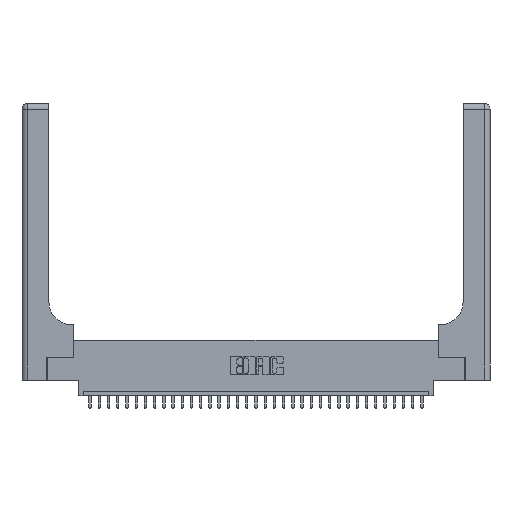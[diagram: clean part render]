
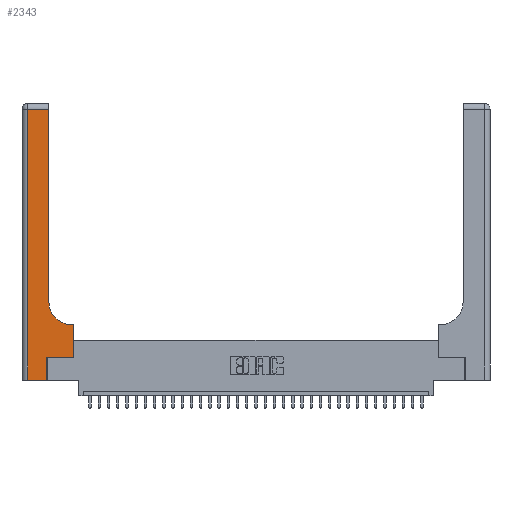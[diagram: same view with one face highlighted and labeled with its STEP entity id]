
A CAD part, top view. The second image highlights one B-rep face of the part: STEP entity #2343.
In plain terms, the highlighted planar face has unit normal (0, 0, 1).
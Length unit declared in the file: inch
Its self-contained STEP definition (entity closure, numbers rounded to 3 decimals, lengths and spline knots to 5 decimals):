
#44 = DIRECTION ( 'NONE',  ( 1., 0., 0. ) ) ;
#453 = CARTESIAN_POINT ( 'NONE',  ( 0.2915, 0.6, 0.37 ) ) ;
#1521 = CARTESIAN_POINT ( 'NONE',  ( 0.5415, 0.85, 0.37 ) ) ;
#1815 = CARTESIAN_POINT ( 'NONE',  ( 0.06, 0., 0.37 ) ) ;
#1894 = DIRECTION ( 'NONE',  ( -1., 0., 0. ) ) ;
#2343 = ADVANCED_FACE ( 'NONE', ( #16079 ), #14926, .F. ) ;
#3345 = LINE ( 'NONE', #25797, #30321 ) ;
#5041 = VECTOR ( 'NONE', #14339, 39.37008 ) ;
#7124 = CARTESIAN_POINT ( 'NONE',  ( 0., 3., 0.37 ) ) ;
#7557 = CARTESIAN_POINT ( 'NONE',  ( 0.06, 3., 0.37 ) ) ;
#7949 = CARTESIAN_POINT ( 'NONE',  ( 0.269, 0., 0.37 ) ) ;
#8164 = EDGE_CURVE ( 'NONE', #15728, #21541, #27175, .T. ) ;
#8396 = CARTESIAN_POINT ( 'NONE',  ( 0.2915, 0.85, 0.37 ) ) ;
#10462 = AXIS2_PLACEMENT_3D ( 'NONE', #1521, #33048, #30664 ) ;
#10763 = EDGE_CURVE ( 'NONE', #21541, #19920, #27013, .T. ) ;
#11228 = EDGE_LOOP ( 'NONE', ( #24741, #26455, #27806, #13317, #22384, #18113, #16411, #21456, #15497 ) ) ;
#11329 = DIRECTION ( 'NONE',  ( -1., 0., 0. ) ) ;
#11653 = VERTEX_POINT ( 'NONE', #29360 ) ;
#12967 = VECTOR ( 'NONE', #33252, 39.37008 ) ;
#13317 = ORIENTED_EDGE ( 'NONE', *, *, #8164, .T. ) ;
#14166 = CARTESIAN_POINT ( 'NONE',  ( 0.5415, 0.6, 0.37 ) ) ;
#14339 = DIRECTION ( 'NONE',  ( 1., 0., 0. ) ) ;
#14682 = VECTOR ( 'NONE', #11329, 39.37008 ) ;
#14926 = PLANE ( 'NONE',  #19494 ) ;
#15497 = ORIENTED_EDGE ( 'NONE', *, *, #32342, .T. ) ;
#15711 = DIRECTION ( 'NONE',  ( 0., -1., 0. ) ) ;
#15728 = VERTEX_POINT ( 'NONE', #1815 ) ;
#15775 = VECTOR ( 'NONE', #33637, 39.37008 ) ;
#16079 = FACE_OUTER_BOUND ( 'NONE', #11228, .T. ) ;
#16411 = ORIENTED_EDGE ( 'NONE', *, *, #29779, .T. ) ;
#16461 = EDGE_CURVE ( 'NONE', #25185, #27807, #3345, .T. ) ;
#16769 = VECTOR ( 'NONE', #26402, 39.37008 ) ;
#17730 = CARTESIAN_POINT ( 'NONE',  ( 0.269, 0., 0.37 ) ) ;
#18113 = ORIENTED_EDGE ( 'NONE', *, *, #22269, .T. ) ;
#18917 = VERTEX_POINT ( 'NONE', #21245 ) ;
#18991 = LINE ( 'NONE', #27727, #5041 ) ;
#19330 = EDGE_CURVE ( 'NONE', #29041, #15728, #31767, .T. ) ;
#19358 = CIRCLE ( 'NONE', #10462, 0.25 ) ;
#19494 = AXIS2_PLACEMENT_3D ( 'NONE', #7124, #27985, #1894 ) ;
#19920 = VERTEX_POINT ( 'NONE', #25752 ) ;
#20767 = CARTESIAN_POINT ( 'NONE',  ( 0., 0., 0.37 ) ) ;
#21245 = CARTESIAN_POINT ( 'NONE',  ( 0.5585, 0.25, 0.37 ) ) ;
#21456 = ORIENTED_EDGE ( 'NONE', *, *, #29005, .T. ) ;
#21541 = VERTEX_POINT ( 'NONE', #7949 ) ;
#21593 = LINE ( 'NONE', #28043, #12967 ) ;
#22269 = EDGE_CURVE ( 'NONE', #19920, #18917, #18991, .T. ) ;
#22275 = VECTOR ( 'NONE', #44, 39.37008 ) ;
#22384 = ORIENTED_EDGE ( 'NONE', *, *, #10763, .T. ) ;
#22722 = LINE ( 'NONE', #33199, #15775 ) ;
#24058 = VECTOR ( 'NONE', #15711, 39.37008 ) ;
#24124 = LINE ( 'NONE', #453, #14682 ) ;
#24741 = ORIENTED_EDGE ( 'NONE', *, *, #16461, .T. ) ;
#25185 = VERTEX_POINT ( 'NONE', #8396 ) ;
#25752 = CARTESIAN_POINT ( 'NONE',  ( 0.269, 0.25, 0.37 ) ) ;
#25797 = CARTESIAN_POINT ( 'NONE',  ( 0.2915, 3., 0.37 ) ) ;
#26402 = DIRECTION ( 'NONE',  ( 0., 1., 0. ) ) ;
#26455 = ORIENTED_EDGE ( 'NONE', *, *, #33680, .T. ) ;
#26480 = VERTEX_POINT ( 'NONE', #14166 ) ;
#26555 = CARTESIAN_POINT ( 'NONE',  ( 0.06, 2.94, 0.37 ) ) ;
#27013 = LINE ( 'NONE', #17730, #16769 ) ;
#27175 = LINE ( 'NONE', #20767, #22275 ) ;
#27727 = CARTESIAN_POINT ( 'NONE',  ( 0.269, 0.25, 0.37 ) ) ;
#27806 = ORIENTED_EDGE ( 'NONE', *, *, #19330, .T. ) ;
#27807 = VERTEX_POINT ( 'NONE', #28806 ) ;
#27985 = DIRECTION ( 'NONE',  ( 0., 0., -1. ) ) ;
#28043 = CARTESIAN_POINT ( 'NONE',  ( 0.5585, 0.25, 0.37 ) ) ;
#28806 = CARTESIAN_POINT ( 'NONE',  ( 0.2915, 2.94, 0.37 ) ) ;
#29005 = EDGE_CURVE ( 'NONE', #11653, #26480, #24124, .T. ) ;
#29041 = VERTEX_POINT ( 'NONE', #26555 ) ;
#29360 = CARTESIAN_POINT ( 'NONE',  ( 0.5585, 0.6, 0.37 ) ) ;
#29779 = EDGE_CURVE ( 'NONE', #18917, #11653, #21593, .T. ) ;
#30321 = VECTOR ( 'NONE', #33625, 39.37008 ) ;
#30664 = DIRECTION ( 'NONE',  ( 1., 0., 0. ) ) ;
#31767 = LINE ( 'NONE', #7557, #24058 ) ;
#32342 = EDGE_CURVE ( 'NONE', #26480, #25185, #19358, .T. ) ;
#33048 = DIRECTION ( 'NONE',  ( 0., 0., -1. ) ) ;
#33199 = CARTESIAN_POINT ( 'NONE',  ( 0., 2.94, 0.37 ) ) ;
#33252 = DIRECTION ( 'NONE',  ( 0., 1., 0. ) ) ;
#33625 = DIRECTION ( 'NONE',  ( 0., 1., 0. ) ) ;
#33637 = DIRECTION ( 'NONE',  ( -1., 0., 0. ) ) ;
#33680 = EDGE_CURVE ( 'NONE', #27807, #29041, #22722, .T. ) ;
